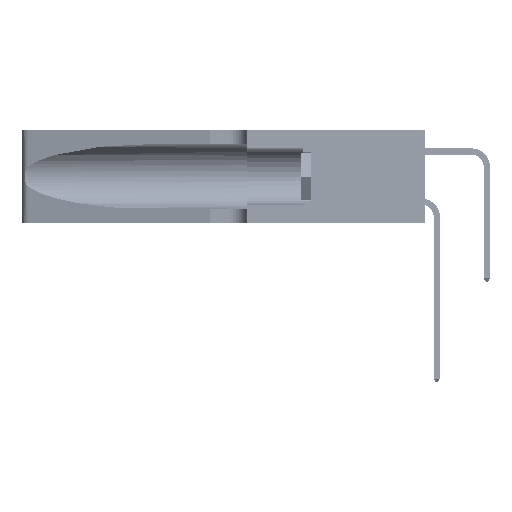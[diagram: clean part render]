
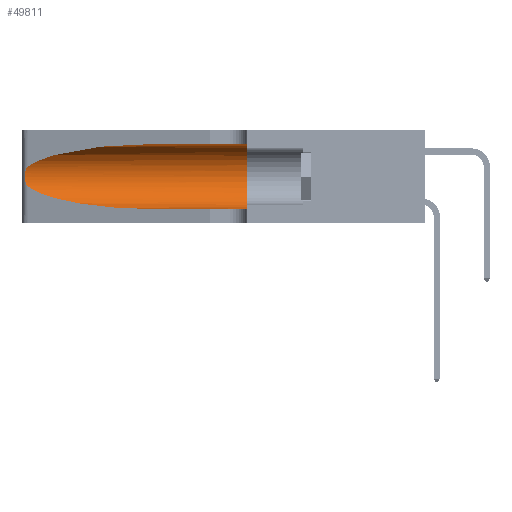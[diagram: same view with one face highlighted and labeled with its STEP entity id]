
A CAD part, left-side view. The second image highlights one B-rep face of the part: STEP entity #49811.
In plain terms, the highlighted cylindrical face has radius 3.308 mm (diameter 6.617 mm), a partial arc.
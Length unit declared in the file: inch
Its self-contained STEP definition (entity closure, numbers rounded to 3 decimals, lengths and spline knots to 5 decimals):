
#206 = DIRECTION ( 'NONE',  ( 0., 0., -1. ) ) ;
#528 = FACE_OUTER_BOUND ( 'NONE', #41709, .T. ) ;
#1281 = CARTESIAN_POINT ( 'NONE',  ( 0.26075, 1.23896, 0.178 ) ) ;
#2676 = VERTEX_POINT ( 'NONE', #48825 ) ;
#2783 = VERTEX_POINT ( 'NONE', #49557 ) ;
#3433 = CARTESIAN_POINT ( 'NONE',  ( 0.18966, 0.96281, 0.31525 ) ) ;
#5510 = CARTESIAN_POINT ( 'NONE',  ( 0.25856, 1.23593, 0.16098 ) ) ;
#7540 = VECTOR ( 'NONE', #13040, 39.37008 ) ;
#7602 = CARTESIAN_POINT ( 'NONE',  ( 0.1305, 0.72297, 0.05475 ) ) ;
#7664 = CARTESIAN_POINT ( 'NONE',  ( 0.2373, 1.15595, 0.28018 ) ) ;
#9694 = EDGE_CURVE ( 'NONE', #2783, #9763, #28174, .T. ) ;
#9737 = CARTESIAN_POINT ( 'NONE',  ( 0.25639, 1.23186, 0.15144 ) ) ;
#9763 = VERTEX_POINT ( 'NONE', #52239 ) ;
#10745 = ORIENTED_EDGE ( 'NONE', *, *, #28725, .T. ) ;
#12679 =( BOUNDED_CURVE ( )  B_SPLINE_CURVE ( 3, ( #35869, #40120, #14861, #44344 ),
 .UNSPECIFIED., .F., .F. ) 
 B_SPLINE_CURVE_WITH_KNOTS ( ( 4, 4 ),
 ( 3.44316, 4.71239 ),
 .UNSPECIFIED. ) 
 CURVE ( )  GEOMETRIC_REPRESENTATION_ITEM ( )  RATIONAL_B_SPLINE_CURVE ( ( 1., 0.87, 0.87, 1. ) ) 
 REPRESENTATION_ITEM ( '' )  );
#13040 = DIRECTION ( 'NONE',  ( 0., -1., 0. ) ) ;
#13094 = ORIENTED_EDGE ( 'NONE', *, *, #45696, .F. ) ;
#13988 = CARTESIAN_POINT ( 'NONE',  ( 0.25487, 1.22718, 0.14631 ) ) ;
#14861 = CARTESIAN_POINT ( 'NONE',  ( 0.18966, 0.96281, 0.05475 ) ) ;
#17153 = DIRECTION ( 'NONE',  ( 0., -1., 0. ) ) ;
#17513 = CARTESIAN_POINT ( 'NONE',  ( 0.1305, 0.35, 0.185 ) ) ;
#17587 = CARTESIAN_POINT ( 'NONE',  ( 0.1305, 0.35, 0.31525 ) ) ;
#18077 = CARTESIAN_POINT ( 'NONE',  ( 0.25639, 1.23184, 0.21858 ) ) ;
#18337 = DIRECTION ( 'NONE',  ( 0., -1., 0. ) ) ;
#18803 = LINE ( 'NONE', #29421, #7540 ) ;
#20258 = VERTEX_POINT ( 'NONE', #52557 ) ;
#21609 = CYLINDRICAL_SURFACE ( 'NONE', #45412, 0.13025 ) ;
#21718 = DIRECTION ( 'NONE',  ( 0., 0., 1. ) ) ;
#22280 = CARTESIAN_POINT ( 'NONE',  ( 0.25854, 1.2359, 0.20912 ) ) ;
#24040 = VERTEX_POINT ( 'NONE', #7602 ) ;
#24301 = VERTEX_POINT ( 'NONE', #17587 ) ;
#25831 =( BOUNDED_CURVE ( )  B_SPLINE_CURVE ( 3, ( #32928, #3433, #7664, #37168 ),
 .UNSPECIFIED., .F., .F. ) 
 B_SPLINE_CURVE_WITH_KNOTS ( ( 4, 4 ),
 ( 1.5708, 2.84003 ),
 .UNSPECIFIED. ) 
 CURVE ( )  GEOMETRIC_REPRESENTATION_ITEM ( )  RATIONAL_B_SPLINE_CURVE ( ( 1., 0.87, 0.87, 1. ) ) 
 REPRESENTATION_ITEM ( '' )  );
#26315 = CARTESIAN_POINT ( 'NONE',  ( 0.25487, 1.22718, 0.22369 ) ) ;
#26495 = CARTESIAN_POINT ( 'NONE',  ( 0.26075, 1.23896, 0.19203 ) ) ;
#28174 = B_SPLINE_CURVE_WITH_KNOTS ( 'NONE', 3,
 ( #26315, #30571, #18077, #47508, #22280, #51704, #26495, #1281, #30750, #5510, #35012, #9737, #39255, #13988 ),
 .UNSPECIFIED., .F., .F.,
 ( 4, 2, 2, 2, 2, 2, 4 ),
 ( 0., 0.00027, 0.00053, 0.00107, 0.0016, 0.00187, 0.00214 ),
 .UNSPECIFIED. ) ;
#28217 = EDGE_CURVE ( 'NONE', #9763, #24040, #12679, .T. ) ;
#28725 = EDGE_CURVE ( 'NONE', #24040, #2676, #42836, .T. ) ;
#29421 = CARTESIAN_POINT ( 'NONE',  ( 0.1305, 1.61858, 0.31525 ) ) ;
#29872 = EDGE_CURVE ( 'NONE', #24301, #2676, #33455, .T. ) ;
#30571 = CARTESIAN_POINT ( 'NONE',  ( 0.25555, 1.22994, 0.2215 ) ) ;
#30750 = CARTESIAN_POINT ( 'NONE',  ( 0.26017, 1.23833, 0.17102 ) ) ;
#32605 = ORIENTED_EDGE ( 'NONE', *, *, #28217, .T. ) ;
#32617 = ORIENTED_EDGE ( 'NONE', *, *, #35695, .T. ) ;
#32928 = CARTESIAN_POINT ( 'NONE',  ( 0.1305, 0.72297, 0.31525 ) ) ;
#33455 = CIRCLE ( 'NONE', #40217, 0.13025 ) ;
#34320 = ORIENTED_EDGE ( 'NONE', *, *, #9694, .T. ) ;
#35012 = CARTESIAN_POINT ( 'NONE',  ( 0.25789, 1.23486, 0.15765 ) ) ;
#35695 = EDGE_CURVE ( 'NONE', #20258, #2783, #25831, .T. ) ;
#35869 = CARTESIAN_POINT ( 'NONE',  ( 0.25487, 1.22718, 0.14631 ) ) ;
#37168 = CARTESIAN_POINT ( 'NONE',  ( 0.25487, 1.22718, 0.22369 ) ) ;
#39255 = CARTESIAN_POINT ( 'NONE',  ( 0.25555, 1.22993, 0.14849 ) ) ;
#40120 = CARTESIAN_POINT ( 'NONE',  ( 0.2373, 1.15595, 0.08982 ) ) ;
#40217 = AXIS2_PLACEMENT_3D ( 'NONE', #17513, #46947, #21718 ) ;
#41709 = EDGE_LOOP ( 'NONE', ( #32617, #34320, #32605, #10745, #43864, #13094 ) ) ;
#42390 = CARTESIAN_POINT ( 'NONE',  ( 0.1305, 1.61858, 0.185 ) ) ;
#42836 = LINE ( 'NONE', #43565, #44137 ) ;
#43565 = CARTESIAN_POINT ( 'NONE',  ( 0.1305, 1.61858, 0.05475 ) ) ;
#43864 = ORIENTED_EDGE ( 'NONE', *, *, #29872, .F. ) ;
#44137 = VECTOR ( 'NONE', #18337, 39.37008 ) ;
#44344 = CARTESIAN_POINT ( 'NONE',  ( 0.1305, 0.72297, 0.05475 ) ) ;
#45412 = AXIS2_PLACEMENT_3D ( 'NONE', #42390, #17153, #206 ) ;
#45696 = EDGE_CURVE ( 'NONE', #20258, #24301, #18803, .T. ) ;
#46947 = DIRECTION ( 'NONE',  ( 0., 1., 0. ) ) ;
#47508 = CARTESIAN_POINT ( 'NONE',  ( 0.25787, 1.23484, 0.2124 ) ) ;
#48825 = CARTESIAN_POINT ( 'NONE',  ( 0.1305, 0.35, 0.05475 ) ) ;
#49557 = CARTESIAN_POINT ( 'NONE',  ( 0.25487, 1.22718, 0.22369 ) ) ;
#49811 = ADVANCED_FACE ( 'NONE', ( #528 ), #21609, .F. ) ;
#51704 = CARTESIAN_POINT ( 'NONE',  ( 0.26018, 1.23835, 0.19895 ) ) ;
#52239 = CARTESIAN_POINT ( 'NONE',  ( 0.25487, 1.22718, 0.14631 ) ) ;
#52557 = CARTESIAN_POINT ( 'NONE',  ( 0.1305, 0.72297, 0.31525 ) ) ;
